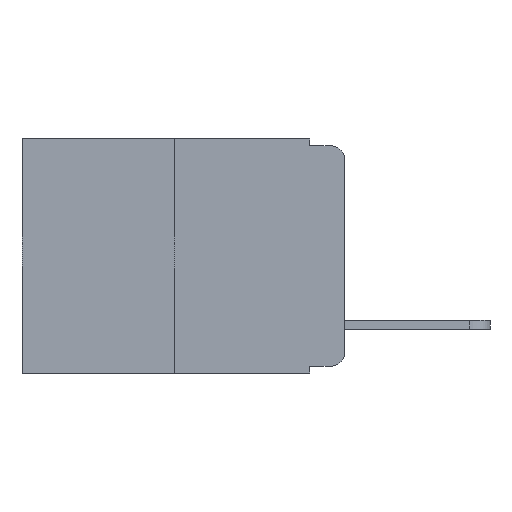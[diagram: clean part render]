
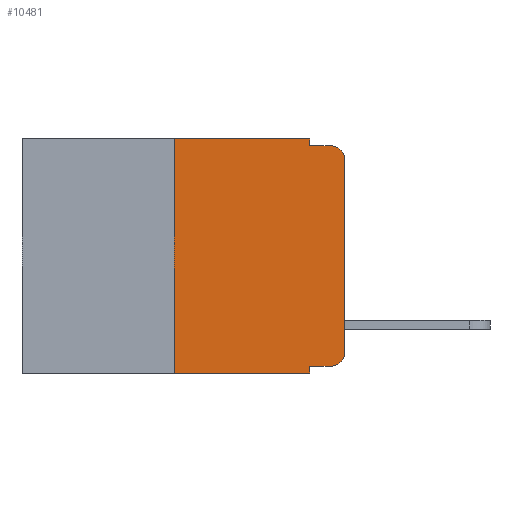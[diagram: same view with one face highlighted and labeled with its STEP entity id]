
A CAD part, left-side view. The second image highlights one B-rep face of the part: STEP entity #10481.
In plain terms, the highlighted planar face has unit normal (-1, 0, 0).
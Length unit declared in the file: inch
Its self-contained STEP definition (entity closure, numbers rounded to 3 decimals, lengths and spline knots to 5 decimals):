
#181 = DIRECTION ( 'NONE',  ( 0., -1., 0. ) ) ;
#358 = VECTOR ( 'NONE', #7333, 39.37008 ) ;
#364 = ORIENTED_EDGE ( 'NONE', *, *, #1368, .T. ) ;
#464 = EDGE_CURVE ( 'NONE', #11294, #10568, #7058, .T. ) ;
#499 = VECTOR ( 'NONE', #7308, 39.37008 ) ;
#544 = CARTESIAN_POINT ( 'NONE',  ( 0., 0.02, -0.333 ) ) ;
#894 = EDGE_LOOP ( 'NONE', ( #1536, #364, #7127, #2858, #6776, #10007, #11203, #11525, #6386, #3131 ) ) ;
#937 = VECTOR ( 'NONE', #3404, 39.37008 ) ;
#1096 = VERTEX_POINT ( 'NONE', #4949 ) ;
#1254 = DIRECTION ( 'NONE',  ( 0., 0., -1. ) ) ;
#1271 = CARTESIAN_POINT ( 'NONE',  ( 0., 0.473, -0.343 ) ) ;
#1368 = EDGE_CURVE ( 'NONE', #2066, #9761, #4952, .T. ) ;
#1536 = ORIENTED_EDGE ( 'NONE', *, *, #1867, .T. ) ;
#1584 = DIRECTION ( 'NONE',  ( -1., 0., 0. ) ) ;
#1668 = DIRECTION ( 'NONE',  ( 0., 0., 1. ) ) ;
#1706 = EDGE_CURVE ( 'NONE', #6464, #4128, #10256, .T. ) ;
#1867 = EDGE_CURVE ( 'NONE', #2663, #2066, #3071, .T. ) ;
#1971 = CARTESIAN_POINT ( 'NONE',  ( 0., 0.051, -0.333 ) ) ;
#2066 = VERTEX_POINT ( 'NONE', #4815 ) ;
#2579 = CARTESIAN_POINT ( 'NONE',  ( 0., 0.25, 0. ) ) ;
#2663 = VERTEX_POINT ( 'NONE', #7648 ) ;
#2858 = ORIENTED_EDGE ( 'NONE', *, *, #8551, .F. ) ;
#2944 = LINE ( 'NONE', #5906, #937 ) ;
#3071 = LINE ( 'NONE', #5471, #499 ) ;
#3100 = CARTESIAN_POINT ( 'NONE',  ( 0., 0.051, 0. ) ) ;
#3131 = ORIENTED_EDGE ( 'NONE', *, *, #6840, .T. ) ;
#3237 = AXIS2_PLACEMENT_3D ( 'NONE', #4284, #1584, #7979 ) ;
#3404 = DIRECTION ( 'NONE',  ( 0., -1., 0. ) ) ;
#3575 = DIRECTION ( 'NONE',  ( 0., 0., -1. ) ) ;
#3875 = CARTESIAN_POINT ( 'NONE',  ( 0., 0.473, 0. ) ) ;
#4128 = VERTEX_POINT ( 'NONE', #544 ) ;
#4195 = VECTOR ( 'NONE', #1254, 39.37008 ) ;
#4235 = CARTESIAN_POINT ( 'NONE',  ( 0., 0.051, -0.333 ) ) ;
#4281 = CARTESIAN_POINT ( 'NONE',  ( 0., 0.02, -0.01 ) ) ;
#4284 = CARTESIAN_POINT ( 'NONE',  ( 0., 0.02, -0.313 ) ) ;
#4313 = VECTOR ( 'NONE', #181, 39.37008 ) ;
#4408 = CARTESIAN_POINT ( 'NONE',  ( 0., 0.02, -0.03 ) ) ;
#4414 = VECTOR ( 'NONE', #1668, 39.37008 ) ;
#4743 = AXIS2_PLACEMENT_3D ( 'NONE', #3875, #7502, #4798 ) ;
#4798 = DIRECTION ( 'NONE',  ( 0., 0., -1. ) ) ;
#4815 = CARTESIAN_POINT ( 'NONE',  ( 0., 0., -0.03 ) ) ;
#4842 = PLANE ( 'NONE',  #4743 ) ;
#4949 = CARTESIAN_POINT ( 'NONE',  ( 0., 0.051, 0. ) ) ;
#4952 = CIRCLE ( 'NONE', #9854, 0.02 ) ;
#5397 = EDGE_CURVE ( 'NONE', #6464, #10568, #6692, .T. ) ;
#5419 = CARTESIAN_POINT ( 'NONE',  ( 0., 0.25, 0. ) ) ;
#5471 = CARTESIAN_POINT ( 'NONE',  ( 0., 0., 0. ) ) ;
#5512 = EDGE_CURVE ( 'NONE', #10264, #9761, #2944, .T. ) ;
#5906 = CARTESIAN_POINT ( 'NONE',  ( 0., 0.051, -0.01 ) ) ;
#5995 = CARTESIAN_POINT ( 'NONE',  ( 0., 0.051, -0.01 ) ) ;
#6055 = CARTESIAN_POINT ( 'NONE',  ( 0., 0.051, -0.343 ) ) ;
#6274 = DIRECTION ( 'NONE',  ( 0., 0., -1. ) ) ;
#6386 = ORIENTED_EDGE ( 'NONE', *, *, #1706, .T. ) ;
#6464 = VERTEX_POINT ( 'NONE', #4235 ) ;
#6692 = LINE ( 'NONE', #3100, #4195 ) ;
#6776 = ORIENTED_EDGE ( 'NONE', *, *, #9342, .F. ) ;
#6840 = EDGE_CURVE ( 'NONE', #4128, #2663, #8755, .T. ) ;
#7058 = LINE ( 'NONE', #1271, #4313 ) ;
#7127 = ORIENTED_EDGE ( 'NONE', *, *, #5512, .F. ) ;
#7308 = DIRECTION ( 'NONE',  ( 0., 0., 1. ) ) ;
#7333 = DIRECTION ( 'NONE',  ( 0., -1., 0. ) ) ;
#7446 = LINE ( 'NONE', #8142, #10865 ) ;
#7502 = DIRECTION ( 'NONE',  ( 1., 0., 0. ) ) ;
#7648 = CARTESIAN_POINT ( 'NONE',  ( 0., 0., -0.313 ) ) ;
#7979 = DIRECTION ( 'NONE',  ( 0., 0., -1. ) ) ;
#8031 = DIRECTION ( 'NONE',  ( 0., -1., 0. ) ) ;
#8135 = LINE ( 'NONE', #2579, #4414 ) ;
#8142 = CARTESIAN_POINT ( 'NONE',  ( 0., 0.473, 0. ) ) ;
#8551 = EDGE_CURVE ( 'NONE', #1096, #10264, #11041, .T. ) ;
#8755 = CIRCLE ( 'NONE', #3237, 0.02 ) ;
#9342 = EDGE_CURVE ( 'NONE', #10104, #1096, #7446, .T. ) ;
#9376 = EDGE_CURVE ( 'NONE', #11294, #10104, #8135, .T. ) ;
#9761 = VERTEX_POINT ( 'NONE', #4281 ) ;
#9854 = AXIS2_PLACEMENT_3D ( 'NONE', #4408, #10820, #6274 ) ;
#10007 = ORIENTED_EDGE ( 'NONE', *, *, #9376, .F. ) ;
#10104 = VERTEX_POINT ( 'NONE', #5419 ) ;
#10256 = LINE ( 'NONE', #1971, #358 ) ;
#10264 = VERTEX_POINT ( 'NONE', #5995 ) ;
#10481 = ADVANCED_FACE ( 'NONE', ( #10704 ), #4842, .F. ) ;
#10568 = VERTEX_POINT ( 'NONE', #6055 ) ;
#10685 = CARTESIAN_POINT ( 'NONE',  ( 0., 0.25, -0.343 ) ) ;
#10704 = FACE_OUTER_BOUND ( 'NONE', #894, .T. ) ;
#10820 = DIRECTION ( 'NONE',  ( -1., 0., 0. ) ) ;
#10865 = VECTOR ( 'NONE', #8031, 39.37008 ) ;
#11041 = LINE ( 'NONE', #11807, #11569 ) ;
#11203 = ORIENTED_EDGE ( 'NONE', *, *, #464, .T. ) ;
#11294 = VERTEX_POINT ( 'NONE', #10685 ) ;
#11525 = ORIENTED_EDGE ( 'NONE', *, *, #5397, .F. ) ;
#11569 = VECTOR ( 'NONE', #3575, 39.37008 ) ;
#11807 = CARTESIAN_POINT ( 'NONE',  ( 0., 0.051, 0. ) ) ;
